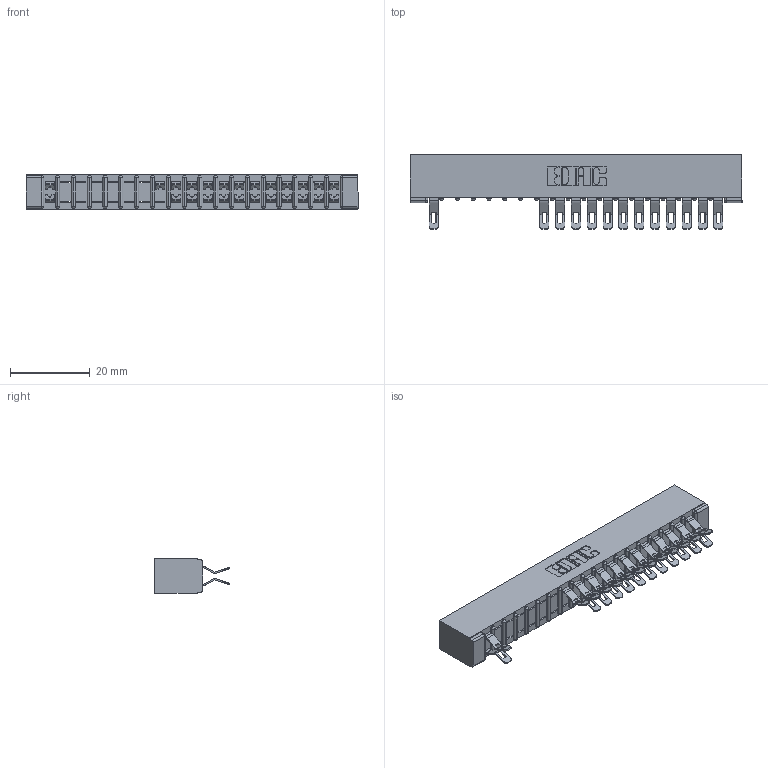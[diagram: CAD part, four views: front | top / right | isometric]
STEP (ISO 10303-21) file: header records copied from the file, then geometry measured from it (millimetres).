
FILE_DESCRIPTION (( 'STEP AP203' ), '1' );
FILE_NAME ('307-038-555-201.STEP', '2018-08-05T11:54:47', ( '' ), ( '' ), 'SwSTEP 2.0', 'SolidWorks 2016', '' );
FILE_SCHEMA (( 'CONFIG_CONTROL_DESIGN' ));
Length unit declared in the file: inch
Products named in the file (3): 307 Part_No Mounting Lugs; 307-290-001_555; 307-038-555-201
Assembly tree (26 placements, depth 2):
  307-038-555-201
    307 Part_No Mounting Lugs
    307-290-001_555  x25
Bounding box: 83.16 x 18.75 x 8.71 mm (x, y, z)
Volume: 5579.1 mm3; surface area: 9585.8 mm2
Topology: 26 solids, 26 shells, 1785 faces, 5240 edges, 3404 vertices
Faces by surface type: plane 994, cylinder 751, sphere 40
Entity records: 19575 total; most frequent: CARTESIAN_POINT 3266, ORIENTED_EDGE 3248, DIRECTION 3202, EDGE_CURVE 1624, LINE 1226, VECTOR 1226, VERTEX_POINT 1052, AXIS2_PLACEMENT_3D 988
